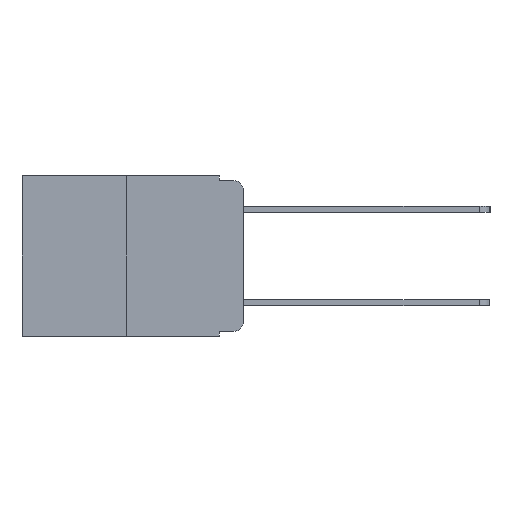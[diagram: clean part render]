
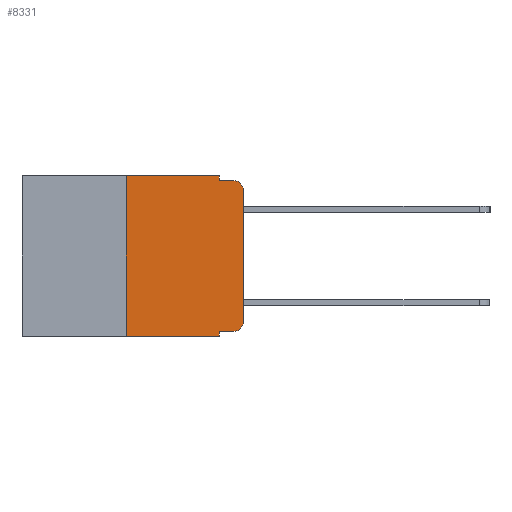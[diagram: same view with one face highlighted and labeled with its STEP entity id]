
A CAD part, left-side view. The second image highlights one B-rep face of the part: STEP entity #8331.
In plain terms, the highlighted planar face has unit normal (-1, 0, 0).
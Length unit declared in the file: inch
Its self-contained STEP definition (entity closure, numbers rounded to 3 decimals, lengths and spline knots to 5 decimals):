
#301 = EDGE_CURVE ( 'NONE', #3579, #13635, #10846, .T. ) ;
#315 = DIRECTION ( 'NONE',  ( 0., 0., 1. ) ) ;
#481 = LINE ( 'NONE', #4329, #6962 ) ;
#562 = ORIENTED_EDGE ( 'NONE', *, *, #12574, .T. ) ;
#716 = CARTESIAN_POINT ( 'NONE',  ( 0., 0., 0. ) ) ;
#752 = CARTESIAN_POINT ( 'NONE',  ( 0., 0.051, -0.333 ) ) ;
#971 = CARTESIAN_POINT ( 'NONE',  ( 0., 0.473, -0.343 ) ) ;
#1079 = ORIENTED_EDGE ( 'NONE', *, *, #3127, .T. ) ;
#1311 = EDGE_CURVE ( 'NONE', #13635, #9835, #4331, .T. ) ;
#1382 = CARTESIAN_POINT ( 'NONE',  ( 0., 0.051, -0.01 ) ) ;
#1565 = LINE ( 'NONE', #11647, #8140 ) ;
#1600 = ORIENTED_EDGE ( 'NONE', *, *, #1311, .F. ) ;
#1889 = FACE_OUTER_BOUND ( 'NONE', #2901, .T. ) ;
#1976 = ORIENTED_EDGE ( 'NONE', *, *, #9360, .F. ) ;
#2121 = VECTOR ( 'NONE', #9729, 39.37008 ) ;
#2170 = DIRECTION ( 'NONE',  ( 0., 0., 1. ) ) ;
#2268 = EDGE_CURVE ( 'NONE', #11892, #9835, #10276, .T. ) ;
#2493 = DIRECTION ( 'NONE',  ( 0., -1., 0. ) ) ;
#2901 = EDGE_LOOP ( 'NONE', ( #1079, #8487, #1600, #9460, #1976, #3004, #4189, #5823, #562, #5603 ) ) ;
#3004 = ORIENTED_EDGE ( 'NONE', *, *, #13894, .F. ) ;
#3127 = EDGE_CURVE ( 'NONE', #10120, #11892, #13911, .T. ) ;
#3579 = VERTEX_POINT ( 'NONE', #6426 ) ;
#3920 = CARTESIAN_POINT ( 'NONE',  ( 0., 0., -0.03 ) ) ;
#4189 = ORIENTED_EDGE ( 'NONE', *, *, #6603, .T. ) ;
#4322 = DIRECTION ( 'NONE',  ( -1., 0., 0. ) ) ;
#4329 = CARTESIAN_POINT ( 'NONE',  ( 0., 0.473, 0. ) ) ;
#4331 = LINE ( 'NONE', #1382, #6569 ) ;
#4443 = DIRECTION ( 'NONE',  ( 1., 0., 0. ) ) ;
#4479 = VECTOR ( 'NONE', #8087, 39.37008 ) ;
#4554 = CARTESIAN_POINT ( 'NONE',  ( 0., 0., -0.313 ) ) ;
#4930 = VERTEX_POINT ( 'NONE', #10870 ) ;
#5037 = DIRECTION ( 'NONE',  ( -1., 0., 0. ) ) ;
#5178 = VECTOR ( 'NONE', #13769, 39.37008 ) ;
#5403 = DIRECTION ( 'NONE',  ( 0., -1., 0. ) ) ;
#5603 = ORIENTED_EDGE ( 'NONE', *, *, #11944, .T. ) ;
#5823 = ORIENTED_EDGE ( 'NONE', *, *, #13225, .F. ) ;
#5852 = CARTESIAN_POINT ( 'NONE',  ( 0., 0.02, -0.01 ) ) ;
#6426 = CARTESIAN_POINT ( 'NONE',  ( 0., 0.051, 0. ) ) ;
#6569 = VECTOR ( 'NONE', #2493, 39.37008 ) ;
#6603 = EDGE_CURVE ( 'NONE', #9380, #8725, #9857, .T. ) ;
#6615 = PLANE ( 'NONE',  #13264 ) ;
#6962 = VECTOR ( 'NONE', #5403, 39.37008 ) ;
#7258 = CARTESIAN_POINT ( 'NONE',  ( 0., 0.051, -0.01 ) ) ;
#7892 = AXIS2_PLACEMENT_3D ( 'NONE', #11335, #5037, #12332 ) ;
#8007 = CIRCLE ( 'NONE', #7892, 0.02 ) ;
#8087 = DIRECTION ( 'NONE',  ( 0., -1., 0. ) ) ;
#8140 = VECTOR ( 'NONE', #315, 39.37008 ) ;
#8166 = LINE ( 'NONE', #8840, #5178 ) ;
#8331 = ADVANCED_FACE ( 'NONE', ( #1889 ), #6615, .F. ) ;
#8487 = ORIENTED_EDGE ( 'NONE', *, *, #2268, .T. ) ;
#8673 = AXIS2_PLACEMENT_3D ( 'NONE', #10671, #4322, #11670 ) ;
#8725 = VERTEX_POINT ( 'NONE', #13052 ) ;
#8840 = CARTESIAN_POINT ( 'NONE',  ( 0., 0.051, -0.333 ) ) ;
#8880 = VERTEX_POINT ( 'NONE', #11253 ) ;
#9114 = VECTOR ( 'NONE', #11975, 39.37008 ) ;
#9360 = EDGE_CURVE ( 'NONE', #4930, #3579, #481, .T. ) ;
#9380 = VERTEX_POINT ( 'NONE', #10635 ) ;
#9460 = ORIENTED_EDGE ( 'NONE', *, *, #301, .F. ) ;
#9729 = DIRECTION ( 'NONE',  ( 0., 0., -1. ) ) ;
#9835 = VERTEX_POINT ( 'NONE', #5852 ) ;
#9857 = LINE ( 'NONE', #971, #4479 ) ;
#10120 = VERTEX_POINT ( 'NONE', #4554 ) ;
#10130 = VERTEX_POINT ( 'NONE', #752 ) ;
#10276 = CIRCLE ( 'NONE', #8673, 0.02 ) ;
#10635 = CARTESIAN_POINT ( 'NONE',  ( 0., 0.25, -0.343 ) ) ;
#10671 = CARTESIAN_POINT ( 'NONE',  ( 0., 0.02, -0.03 ) ) ;
#10777 = CARTESIAN_POINT ( 'NONE',  ( 0., 0.473, 0. ) ) ;
#10846 = LINE ( 'NONE', #11407, #2121 ) ;
#10870 = CARTESIAN_POINT ( 'NONE',  ( 0., 0.25, 0. ) ) ;
#10965 = CARTESIAN_POINT ( 'NONE',  ( 0., 0.051, 0. ) ) ;
#10998 = VECTOR ( 'NONE', #2170, 39.37008 ) ;
#11253 = CARTESIAN_POINT ( 'NONE',  ( 0., 0.02, -0.333 ) ) ;
#11335 = CARTESIAN_POINT ( 'NONE',  ( 0., 0.02, -0.313 ) ) ;
#11407 = CARTESIAN_POINT ( 'NONE',  ( 0., 0.051, 0. ) ) ;
#11647 = CARTESIAN_POINT ( 'NONE',  ( 0., 0.25, 0. ) ) ;
#11670 = DIRECTION ( 'NONE',  ( 0., 0., -1. ) ) ;
#11782 = DIRECTION ( 'NONE',  ( 0., 0., -1. ) ) ;
#11892 = VERTEX_POINT ( 'NONE', #3920 ) ;
#11944 = EDGE_CURVE ( 'NONE', #8880, #10120, #8007, .T. ) ;
#11975 = DIRECTION ( 'NONE',  ( 0., 0., -1. ) ) ;
#12332 = DIRECTION ( 'NONE',  ( 0., 0., -1. ) ) ;
#12574 = EDGE_CURVE ( 'NONE', #10130, #8880, #8166, .T. ) ;
#13052 = CARTESIAN_POINT ( 'NONE',  ( 0., 0.051, -0.343 ) ) ;
#13225 = EDGE_CURVE ( 'NONE', #10130, #8725, #14026, .T. ) ;
#13264 = AXIS2_PLACEMENT_3D ( 'NONE', #10777, #4443, #11782 ) ;
#13635 = VERTEX_POINT ( 'NONE', #7258 ) ;
#13769 = DIRECTION ( 'NONE',  ( 0., -1., 0. ) ) ;
#13894 = EDGE_CURVE ( 'NONE', #9380, #4930, #1565, .T. ) ;
#13911 = LINE ( 'NONE', #716, #10998 ) ;
#14026 = LINE ( 'NONE', #10965, #9114 ) ;
